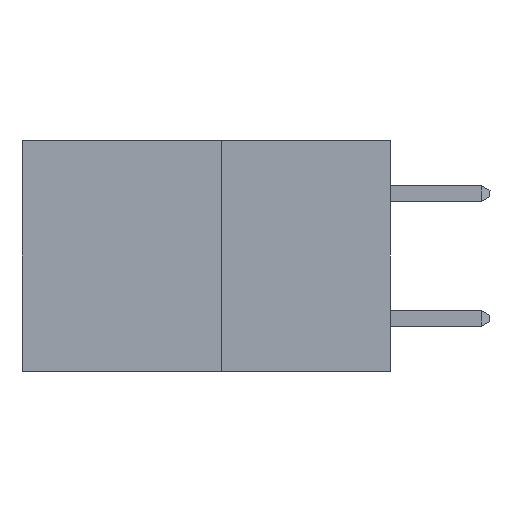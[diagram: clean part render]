
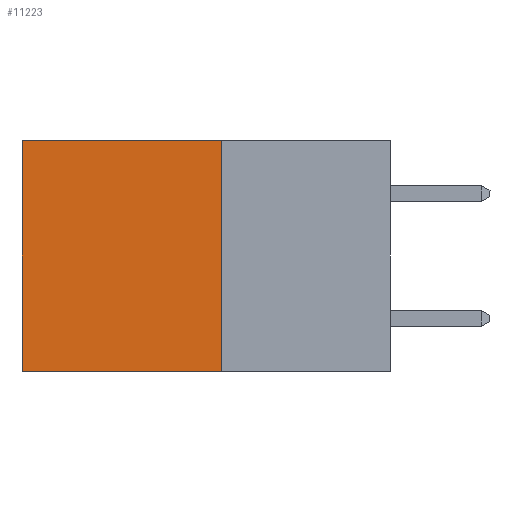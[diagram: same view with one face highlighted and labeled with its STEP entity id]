
A CAD part, left-side view. The second image highlights one B-rep face of the part: STEP entity #11223.
In plain terms, the highlighted planar face has unit normal (-1, 0, 0).
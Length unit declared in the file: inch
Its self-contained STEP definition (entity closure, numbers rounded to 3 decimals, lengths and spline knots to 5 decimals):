
#149 = VECTOR ( 'NONE', #8156, 39.37008 ) ;
#168 = CARTESIAN_POINT ( 'NONE',  ( 0.277, 0.59, -0.37 ) ) ;
#1121 = EDGE_CURVE ( 'NONE', #2628, #8533, #11494, .T. ) ;
#1132 = FACE_OUTER_BOUND ( 'NONE', #5185, .T. ) ;
#1289 = CARTESIAN_POINT ( 'NONE',  ( 0.277, 0.27, -0.37 ) ) ;
#2174 = ORIENTED_EDGE ( 'NONE', *, *, #9843, .T. ) ;
#2216 = CARTESIAN_POINT ( 'NONE',  ( 0.277, 0.27, -0.37 ) ) ;
#2628 = VERTEX_POINT ( 'NONE', #1289 ) ;
#3128 = ORIENTED_EDGE ( 'NONE', *, *, #4022, .T. ) ;
#3898 = CARTESIAN_POINT ( 'NONE',  ( 0.277, 0.59, 0. ) ) ;
#4022 = EDGE_CURVE ( 'NONE', #9367, #13040, #10656, .T. ) ;
#4111 = DIRECTION ( 'NONE',  ( 0., 1., 0. ) ) ;
#4380 = CARTESIAN_POINT ( 'NONE',  ( 0.277, 0.27, 0. ) ) ;
#4852 = AXIS2_PLACEMENT_3D ( 'NONE', #2216, #5695, #13517 ) ;
#5185 = EDGE_LOOP ( 'NONE', ( #2174, #9595, #13273, #3128 ) ) ;
#5695 = DIRECTION ( 'NONE',  ( 1., 0., 0. ) ) ;
#6237 = CARTESIAN_POINT ( 'NONE',  ( 0.277, 0.27, -0.37 ) ) ;
#8156 = DIRECTION ( 'NONE',  ( 0., 0., -1. ) ) ;
#8533 = VERTEX_POINT ( 'NONE', #168 ) ;
#9034 = VECTOR ( 'NONE', #11582, 39.37008 ) ;
#9287 = CARTESIAN_POINT ( 'NONE',  ( 0.277, 0.59, -0.37 ) ) ;
#9367 = VERTEX_POINT ( 'NONE', #14096 ) ;
#9595 = ORIENTED_EDGE ( 'NONE', *, *, #1121, .F. ) ;
#9823 = EDGE_CURVE ( 'NONE', #9367, #2628, #10110, .T. ) ;
#9843 = EDGE_CURVE ( 'NONE', #13040, #8533, #12388, .T. ) ;
#10110 = LINE ( 'NONE', #11540, #149 ) ;
#10656 = LINE ( 'NONE', #4380, #13928 ) ;
#10885 = DIRECTION ( 'NONE',  ( 0., 1., 0. ) ) ;
#11223 = ADVANCED_FACE ( 'NONE', ( #1132 ), #12430, .F. ) ;
#11494 = LINE ( 'NONE', #6237, #13702 ) ;
#11540 = CARTESIAN_POINT ( 'NONE',  ( 0.277, 0.27, -0.37 ) ) ;
#11582 = DIRECTION ( 'NONE',  ( 0., 0., -1. ) ) ;
#12388 = LINE ( 'NONE', #9287, #9034 ) ;
#12430 = PLANE ( 'NONE',  #4852 ) ;
#13040 = VERTEX_POINT ( 'NONE', #3898 ) ;
#13273 = ORIENTED_EDGE ( 'NONE', *, *, #9823, .F. ) ;
#13517 = DIRECTION ( 'NONE',  ( 0., 0., -1. ) ) ;
#13702 = VECTOR ( 'NONE', #10885, 39.37008 ) ;
#13928 = VECTOR ( 'NONE', #4111, 39.37008 ) ;
#14096 = CARTESIAN_POINT ( 'NONE',  ( 0.277, 0.27, 0. ) ) ;
